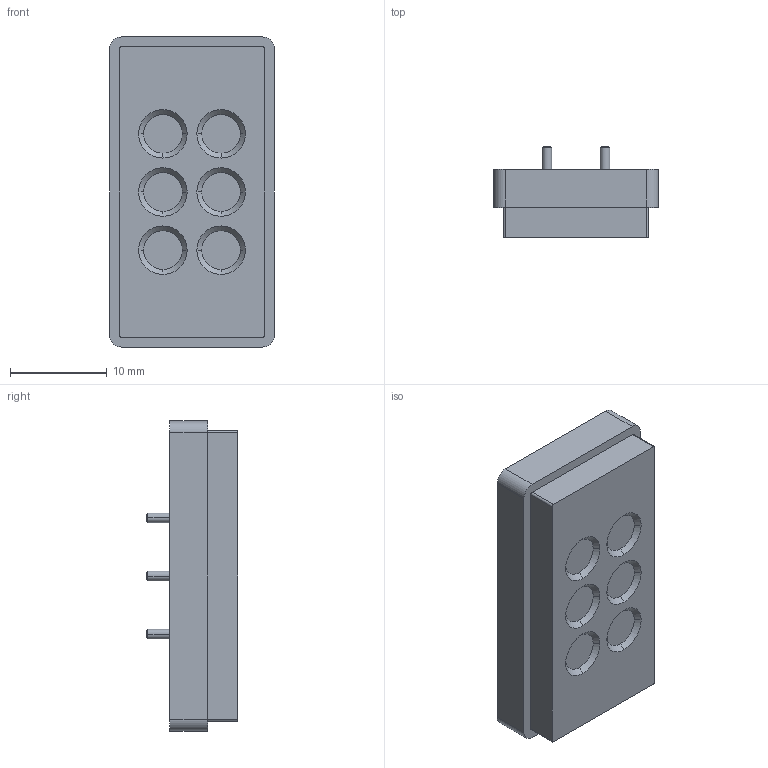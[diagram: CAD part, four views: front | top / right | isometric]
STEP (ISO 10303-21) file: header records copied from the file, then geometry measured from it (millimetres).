
FILE_DESCRIPTION (( 'STEP AP214' ), '1' );
FILE_NAME ('686C06B2260110E.STEP', '2023-04-14T19:58:44', ( '' ), ( '' ), 'SwSTEP 2.0', 'SolidWorks 2020', '' );
FILE_SCHEMA (( 'AUTOMOTIVE_DESIGN' ));
Length unit declared in the file: millimetre
Products named in the file (1): 686C06B2260110E
Bounding box: 17 x 9.4 x 32 mm (x, y, z)
Volume: 2947.2 mm3; surface area: 2752.1 mm2
Topology: 1 solids, 2 shells, 342 faces, 954 edges, 624 vertices
Faces by surface type: plane 224, cylinder 82, cone 36
Entity records: 14132 total; most frequent: CARTESIAN_POINT 1921, ORIENTED_EDGE 1908, DIRECTION 1864, EDGE_CURVE 954, LINE 730, VECTOR 730, VERTEX_POINT 624, AXIS2_PLACEMENT_3D 567
